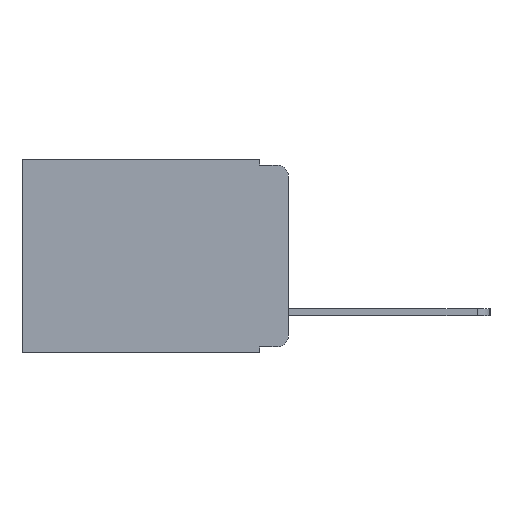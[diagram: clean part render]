
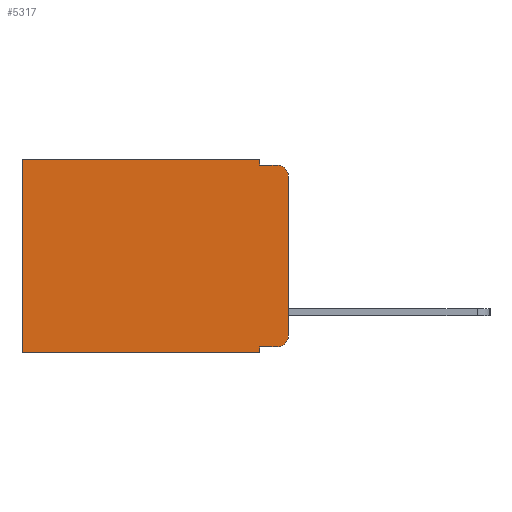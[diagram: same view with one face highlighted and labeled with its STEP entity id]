
A CAD part, left-side view. The second image highlights one B-rep face of the part: STEP entity #5317.
In plain terms, the highlighted planar face has unit normal (-1, 0, 0).
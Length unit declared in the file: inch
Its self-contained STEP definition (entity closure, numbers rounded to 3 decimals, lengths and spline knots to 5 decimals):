
#63 = CARTESIAN_POINT ( 'NONE',  ( 0.298, 0.051, 0. ) ) ;
#151 = VERTEX_POINT ( 'NONE', #63 ) ;
#243 = CARTESIAN_POINT ( 'NONE',  ( 0.298, 0.051, -0.01 ) ) ;
#622 = VECTOR ( 'NONE', #7943, 39.37008 ) ;
#922 = DIRECTION ( 'NONE',  ( 0., 0., -1. ) ) ;
#1044 = VERTEX_POINT ( 'NONE', #11593 ) ;
#1227 = VECTOR ( 'NONE', #10798, 39.37008 ) ;
#1386 = ORIENTED_EDGE ( 'NONE', *, *, #9094, .F. ) ;
#1660 = VERTEX_POINT ( 'NONE', #5458 ) ;
#1858 = EDGE_LOOP ( 'NONE', ( #1386, #6416, #6818, #6855, #2216, #3208, #2737, #4480, #3503, #2616 ) ) ;
#1905 = LINE ( 'NONE', #2014, #8813 ) ;
#2014 = CARTESIAN_POINT ( 'NONE',  ( 0.298, 0.051, -0.333 ) ) ;
#2216 = ORIENTED_EDGE ( 'NONE', *, *, #7971, .T. ) ;
#2435 = AXIS2_PLACEMENT_3D ( 'NONE', #8755, #8798, #4448 ) ;
#2490 = EDGE_CURVE ( 'NONE', #151, #1044, #5010, .T. ) ;
#2616 = ORIENTED_EDGE ( 'NONE', *, *, #8417, .T. ) ;
#2737 = ORIENTED_EDGE ( 'NONE', *, *, #6018, .F. ) ;
#2981 = CIRCLE ( 'NONE', #10483, 0.02 ) ;
#3208 = ORIENTED_EDGE ( 'NONE', *, *, #5721, .T. ) ;
#3309 = DIRECTION ( 'NONE',  ( 0., 0., -1. ) ) ;
#3409 = VERTEX_POINT ( 'NONE', #3794 ) ;
#3503 = ORIENTED_EDGE ( 'NONE', *, *, #7740, .T. ) ;
#3794 = CARTESIAN_POINT ( 'NONE',  ( 0.298, 0.051, -0.343 ) ) ;
#4436 = VECTOR ( 'NONE', #8006, 39.37008 ) ;
#4448 = DIRECTION ( 'NONE',  ( 0., 0., -1. ) ) ;
#4480 = ORIENTED_EDGE ( 'NONE', *, *, #9725, .F. ) ;
#4576 = CARTESIAN_POINT ( 'NONE',  ( 0.298, 0.051, 0. ) ) ;
#4709 = CARTESIAN_POINT ( 'NONE',  ( 0.298, 0., 0. ) ) ;
#4716 = VECTOR ( 'NONE', #3309, 39.37008 ) ;
#5010 = LINE ( 'NONE', #7330, #4716 ) ;
#5317 = ADVANCED_FACE ( 'NONE', ( #10297 ), #8832, .F. ) ;
#5328 = LINE ( 'NONE', #243, #4436 ) ;
#5458 = CARTESIAN_POINT ( 'NONE',  ( 0.298, 0., -0.03 ) ) ;
#5595 = CARTESIAN_POINT ( 'NONE',  ( 0.298, 0.473, 0. ) ) ;
#5721 = EDGE_CURVE ( 'NONE', #6226, #10237, #10534, .T. ) ;
#5814 = AXIS2_PLACEMENT_3D ( 'NONE', #7438, #7346, #7139 ) ;
#5920 = VERTEX_POINT ( 'NONE', #8564 ) ;
#6018 = EDGE_CURVE ( 'NONE', #3409, #10237, #10406, .T. ) ;
#6088 = CARTESIAN_POINT ( 'NONE',  ( 0.298, 0.051, -0.333 ) ) ;
#6161 = CARTESIAN_POINT ( 'NONE',  ( 0.298, 0., 0. ) ) ;
#6226 = VERTEX_POINT ( 'NONE', #5595 ) ;
#6339 = LINE ( 'NONE', #4576, #1227 ) ;
#6416 = ORIENTED_EDGE ( 'NONE', *, *, #6574, .T. ) ;
#6433 = CARTESIAN_POINT ( 'NONE',  ( 0.298, 0.473, -0.343 ) ) ;
#6534 = VECTOR ( 'NONE', #11398, 39.37008 ) ;
#6574 = EDGE_CURVE ( 'NONE', #1660, #5920, #10516, .T. ) ;
#6730 = DIRECTION ( 'NONE',  ( -1., 0., 0. ) ) ;
#6818 = ORIENTED_EDGE ( 'NONE', *, *, #10126, .F. ) ;
#6855 = ORIENTED_EDGE ( 'NONE', *, *, #2490, .F. ) ;
#6989 = VECTOR ( 'NONE', #7246, 39.37008 ) ;
#7139 = DIRECTION ( 'NONE',  ( 0., 0., -1. ) ) ;
#7246 = DIRECTION ( 'NONE',  ( 0., 1., 0. ) ) ;
#7330 = CARTESIAN_POINT ( 'NONE',  ( 0.298, 0.051, 0. ) ) ;
#7346 = DIRECTION ( 'NONE',  ( -1., 0., 0. ) ) ;
#7438 = CARTESIAN_POINT ( 'NONE',  ( 0.298, 0.02, -0.03 ) ) ;
#7740 = EDGE_CURVE ( 'NONE', #10097, #9688, #1905, .T. ) ;
#7795 = VECTOR ( 'NONE', #10100, 39.37008 ) ;
#7943 = DIRECTION ( 'NONE',  ( 0., 0., -1. ) ) ;
#7971 = EDGE_CURVE ( 'NONE', #151, #6226, #9210, .T. ) ;
#8006 = DIRECTION ( 'NONE',  ( 0., -1., 0. ) ) ;
#8201 = CARTESIAN_POINT ( 'NONE',  ( 0.298, 0.02, -0.333 ) ) ;
#8417 = EDGE_CURVE ( 'NONE', #9688, #10047, #2981, .T. ) ;
#8564 = CARTESIAN_POINT ( 'NONE',  ( 0.298, 0.02, -0.01 ) ) ;
#8755 = CARTESIAN_POINT ( 'NONE',  ( 0.298, 0., 0. ) ) ;
#8798 = DIRECTION ( 'NONE',  ( 1., 0., 0. ) ) ;
#8813 = VECTOR ( 'NONE', #9466, 39.37008 ) ;
#8832 = PLANE ( 'NONE',  #2435 ) ;
#9094 = EDGE_CURVE ( 'NONE', #1660, #10047, #10358, .T. ) ;
#9210 = LINE ( 'NONE', #6161, #6534 ) ;
#9466 = DIRECTION ( 'NONE',  ( 0., -1., 0. ) ) ;
#9688 = VERTEX_POINT ( 'NONE', #8201 ) ;
#9725 = EDGE_CURVE ( 'NONE', #10097, #3409, #6339, .T. ) ;
#10047 = VERTEX_POINT ( 'NONE', #11329 ) ;
#10097 = VERTEX_POINT ( 'NONE', #6088 ) ;
#10100 = DIRECTION ( 'NONE',  ( 0., 0., -1. ) ) ;
#10126 = EDGE_CURVE ( 'NONE', #1044, #5920, #5328, .T. ) ;
#10237 = VERTEX_POINT ( 'NONE', #6433 ) ;
#10297 = FACE_OUTER_BOUND ( 'NONE', #1858, .T. ) ;
#10358 = LINE ( 'NONE', #4709, #7795 ) ;
#10406 = LINE ( 'NONE', #11042, #6989 ) ;
#10432 = CARTESIAN_POINT ( 'NONE',  ( 0.298, 0.473, 0. ) ) ;
#10483 = AXIS2_PLACEMENT_3D ( 'NONE', #11904, #6730, #922 ) ;
#10516 = CIRCLE ( 'NONE', #5814, 0.02 ) ;
#10534 = LINE ( 'NONE', #10432, #622 ) ;
#10798 = DIRECTION ( 'NONE',  ( 0., 0., -1. ) ) ;
#11042 = CARTESIAN_POINT ( 'NONE',  ( 0.298, 0., -0.343 ) ) ;
#11329 = CARTESIAN_POINT ( 'NONE',  ( 0.298, 0., -0.313 ) ) ;
#11398 = DIRECTION ( 'NONE',  ( 0., 1., 0. ) ) ;
#11593 = CARTESIAN_POINT ( 'NONE',  ( 0.298, 0.051, -0.01 ) ) ;
#11904 = CARTESIAN_POINT ( 'NONE',  ( 0.298, 0.02, -0.313 ) ) ;
